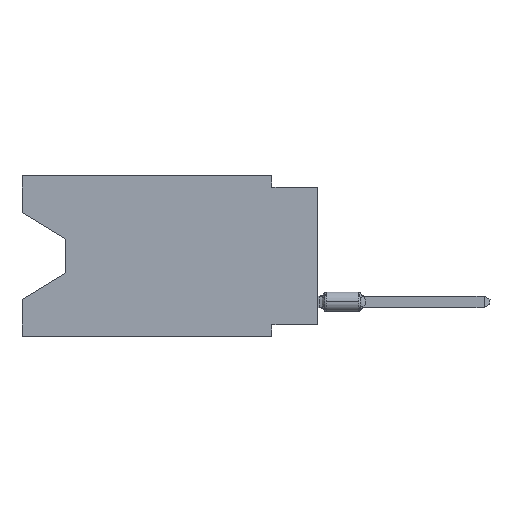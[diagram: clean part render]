
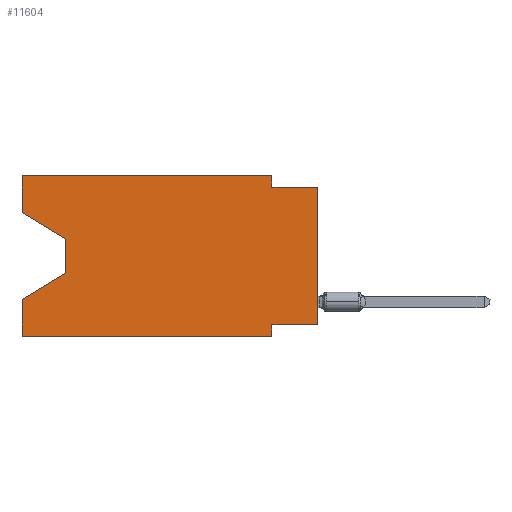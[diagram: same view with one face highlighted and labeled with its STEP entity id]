
A CAD part, left-side view. The second image highlights one B-rep face of the part: STEP entity #11604.
In plain terms, the highlighted planar face has unit normal (-1, 0, 0).
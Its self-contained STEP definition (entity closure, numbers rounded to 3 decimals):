
#150 = ORIENTED_EDGE ( 'NONE', *, *, #3893, .T. ) ;
#323 = EDGE_CURVE ( 'NONE', #5067, #23728, #24081, .T. ) ;
#409 = DIRECTION ( 'NONE',  ( 0., 0., -1. ) ) ;
#508 = EDGE_CURVE ( 'NONE', #20513, #23807, #7221, .T. ) ;
#743 = DIRECTION ( 'NONE',  ( 0., 0., 1. ) ) ;
#834 = VECTOR ( 'NONE', #23185, 1000. ) ;
#1469 = CARTESIAN_POINT ( 'NONE',  ( 0., 16.383, 0. ) ) ;
#1884 = DIRECTION ( 'NONE',  ( 1., 0., 0. ) ) ;
#1905 = CARTESIAN_POINT ( 'NONE',  ( 0., 13.97, -5.385 ) ) ;
#1940 = DIRECTION ( 'NONE',  ( 0., -0.855, -0.519 ) ) ;
#2269 = ORIENTED_EDGE ( 'NONE', *, *, #20388, .F. ) ;
#2326 = VECTOR ( 'NONE', #1940, 1000. ) ;
#2593 = CARTESIAN_POINT ( 'NONE',  ( 0., 16.383, 0. ) ) ;
#2840 = LINE ( 'NONE', #2593, #4876 ) ;
#3207 = VERTEX_POINT ( 'NONE', #8267 ) ;
#3375 = CARTESIAN_POINT ( 'NONE',  ( 0., 0., -8.255 ) ) ;
#3452 = PLANE ( 'NONE',  #22681 ) ;
#3619 = LINE ( 'NONE', #3375, #21525 ) ;
#3893 = EDGE_CURVE ( 'NONE', #3207, #6076, #21650, .T. ) ;
#4036 = EDGE_CURVE ( 'NONE', #24953, #10288, #2840, .T. ) ;
#4503 = DIRECTION ( 'NONE',  ( 0., -1., 0. ) ) ;
#4876 = VECTOR ( 'NONE', #12377, 1000. ) ;
#5067 = VERTEX_POINT ( 'NONE', #15598 ) ;
#5665 = ORIENTED_EDGE ( 'NONE', *, *, #8497, .T. ) ;
#5911 = LINE ( 'NONE', #22026, #14361 ) ;
#6076 = VERTEX_POINT ( 'NONE', #20291 ) ;
#6134 = VECTOR ( 'NONE', #409, 1000. ) ;
#6448 = CARTESIAN_POINT ( 'NONE',  ( 0., 0., -0.635 ) ) ;
#6958 = VECTOR ( 'NONE', #18176, 1000. ) ;
#7221 = LINE ( 'NONE', #17148, #834 ) ;
#7461 = VERTEX_POINT ( 'NONE', #25316 ) ;
#7648 = LINE ( 'NONE', #1469, #13985 ) ;
#7799 = EDGE_CURVE ( 'NONE', #18281, #20513, #3619, .T. ) ;
#7933 = VERTEX_POINT ( 'NONE', #6448 ) ;
#8267 = CARTESIAN_POINT ( 'NONE',  ( 0., 13.97, -3.505 ) ) ;
#8497 = EDGE_CURVE ( 'NONE', #18281, #7933, #18390, .T. ) ;
#8793 = ORIENTED_EDGE ( 'NONE', *, *, #323, .F. ) ;
#9214 = CARTESIAN_POINT ( 'NONE',  ( 0., 16.383, -8.89 ) ) ;
#9338 = DIRECTION ( 'NONE',  ( 0., -1., 0. ) ) ;
#9369 = ORIENTED_EDGE ( 'NONE', *, *, #4036, .F. ) ;
#9462 = EDGE_CURVE ( 'NONE', #12845, #23807, #15680, .T. ) ;
#9509 = CARTESIAN_POINT ( 'NONE',  ( 0., 16.383, -8.89 ) ) ;
#9804 = DIRECTION ( 'NONE',  ( 0., 1., 0. ) ) ;
#9857 = CARTESIAN_POINT ( 'NONE',  ( 0., 2.54, -8.255 ) ) ;
#10041 = DIRECTION ( 'NONE',  ( 0., 0., 1. ) ) ;
#10288 = VERTEX_POINT ( 'NONE', #24019 ) ;
#11239 = ORIENTED_EDGE ( 'NONE', *, *, #16685, .T. ) ;
#11557 = FACE_OUTER_BOUND ( 'NONE', #17762, .T. ) ;
#11604 = ADVANCED_FACE ( 'NONE', ( #11557 ), #3452, .F. ) ;
#11632 = CARTESIAN_POINT ( 'NONE',  ( 0., 16.383, -2.038 ) ) ;
#11953 = DIRECTION ( 'NONE',  ( 0., -1., 0. ) ) ;
#12225 = EDGE_CURVE ( 'NONE', #23728, #7933, #14665, .T. ) ;
#12242 = CARTESIAN_POINT ( 'NONE',  ( 0., 13.97, -3.505 ) ) ;
#12328 = VECTOR ( 'NONE', #11953, 1000. ) ;
#12377 = DIRECTION ( 'NONE',  ( 0., 0., 1. ) ) ;
#12421 = VECTOR ( 'NONE', #4503, 1000. ) ;
#12488 = CARTESIAN_POINT ( 'NONE',  ( 0., 2.54, 0. ) ) ;
#12845 = VERTEX_POINT ( 'NONE', #9214 ) ;
#13076 = VECTOR ( 'NONE', #21765, 1000. ) ;
#13985 = VECTOR ( 'NONE', #9338, 1000. ) ;
#14361 = VECTOR ( 'NONE', #10041, 1000. ) ;
#14665 = LINE ( 'NONE', #20727, #12421 ) ;
#15147 = VECTOR ( 'NONE', #743, 1000. ) ;
#15275 = EDGE_CURVE ( 'NONE', #24953, #3207, #23709, .T. ) ;
#15598 = CARTESIAN_POINT ( 'NONE',  ( 0., 2.54, 0. ) ) ;
#15621 = CARTESIAN_POINT ( 'NONE',  ( 0., 2.54, -0.635 ) ) ;
#15674 = DIRECTION ( 'NONE',  ( 0., 0., -1. ) ) ;
#15680 = LINE ( 'NONE', #9509, #12328 ) ;
#15749 = CARTESIAN_POINT ( 'NONE',  ( 0., 2.54, -8.89 ) ) ;
#15910 = ORIENTED_EDGE ( 'NONE', *, *, #508, .F. ) ;
#16075 = CARTESIAN_POINT ( 'NONE',  ( 0., 0., 0. ) ) ;
#16685 = EDGE_CURVE ( 'NONE', #6076, #7461, #23951, .T. ) ;
#17148 = CARTESIAN_POINT ( 'NONE',  ( 0., 2.54, -8.89 ) ) ;
#17762 = EDGE_LOOP ( 'NONE', ( #24531, #150, #11239, #25290, #19009, #15910, #24327, #5665, #21100, #8793, #2269, #9369 ) ) ;
#18176 = DIRECTION ( 'NONE',  ( 0., 0., -1. ) ) ;
#18281 = VERTEX_POINT ( 'NONE', #19163 ) ;
#18390 = LINE ( 'NONE', #16075, #15147 ) ;
#19009 = ORIENTED_EDGE ( 'NONE', *, *, #9462, .T. ) ;
#19163 = CARTESIAN_POINT ( 'NONE',  ( 0., 0., -8.255 ) ) ;
#19561 = EDGE_CURVE ( 'NONE', #12845, #7461, #5911, .T. ) ;
#20291 = CARTESIAN_POINT ( 'NONE',  ( 0., 13.97, -5.385 ) ) ;
#20388 = EDGE_CURVE ( 'NONE', #10288, #5067, #7648, .T. ) ;
#20513 = VERTEX_POINT ( 'NONE', #9857 ) ;
#20727 = CARTESIAN_POINT ( 'NONE',  ( 0., 0., -0.635 ) ) ;
#21100 = ORIENTED_EDGE ( 'NONE', *, *, #12225, .F. ) ;
#21223 = CARTESIAN_POINT ( 'NONE',  ( 0., 16.383, 0. ) ) ;
#21525 = VECTOR ( 'NONE', #9804, 1000. ) ;
#21650 = LINE ( 'NONE', #12242, #6134 ) ;
#21765 = DIRECTION ( 'NONE',  ( 0., 0.855, -0.519 ) ) ;
#22026 = CARTESIAN_POINT ( 'NONE',  ( 0., 16.383, 0. ) ) ;
#22681 = AXIS2_PLACEMENT_3D ( 'NONE', #21223, #1884, #15674 ) ;
#23185 = DIRECTION ( 'NONE',  ( 0., 0., -1. ) ) ;
#23709 = LINE ( 'NONE', #25391, #2326 ) ;
#23728 = VERTEX_POINT ( 'NONE', #15621 ) ;
#23807 = VERTEX_POINT ( 'NONE', #15749 ) ;
#23951 = LINE ( 'NONE', #1905, #13076 ) ;
#24019 = CARTESIAN_POINT ( 'NONE',  ( 0., 16.383, 0. ) ) ;
#24081 = LINE ( 'NONE', #12488, #6958 ) ;
#24327 = ORIENTED_EDGE ( 'NONE', *, *, #7799, .F. ) ;
#24531 = ORIENTED_EDGE ( 'NONE', *, *, #15275, .T. ) ;
#24953 = VERTEX_POINT ( 'NONE', #11632 ) ;
#25290 = ORIENTED_EDGE ( 'NONE', *, *, #19561, .F. ) ;
#25316 = CARTESIAN_POINT ( 'NONE',  ( 0., 16.383, -6.852 ) ) ;
#25391 = CARTESIAN_POINT ( 'NONE',  ( 0., 16.383, -2.038 ) ) ;
